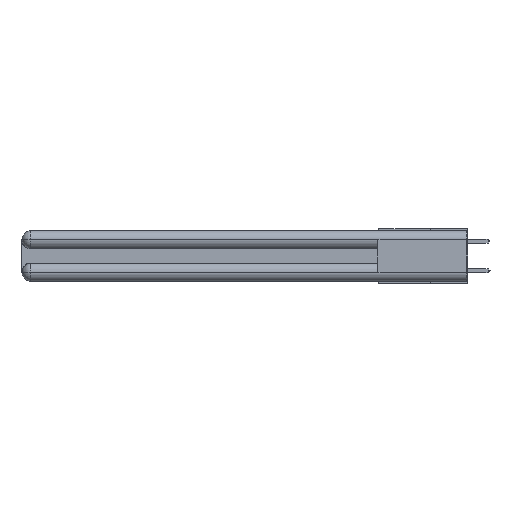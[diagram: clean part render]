
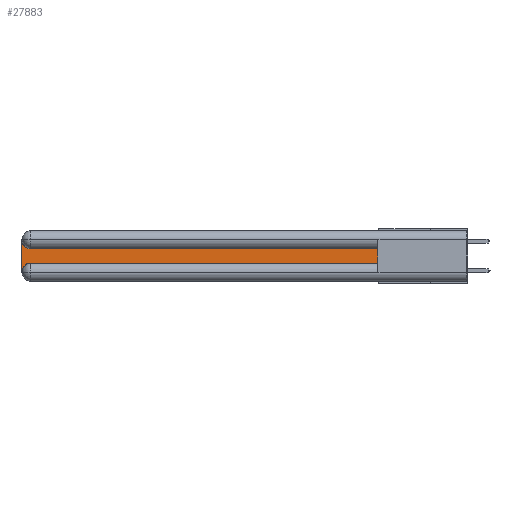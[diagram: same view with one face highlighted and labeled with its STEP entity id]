
A CAD part, left-side view. The second image highlights one B-rep face of the part: STEP entity #27883.
In plain terms, the highlighted planar face has unit normal (-1, 0, 0).
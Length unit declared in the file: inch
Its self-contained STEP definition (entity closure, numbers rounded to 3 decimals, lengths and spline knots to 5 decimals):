
#145 = EDGE_CURVE ( 'NONE', #4539, #19977, #30470, .T. ) ;
#1540 = DIRECTION ( 'NONE',  ( 0., 0., -1. ) ) ;
#2026 = EDGE_CURVE ( 'NONE', #13715, #15117, #4650, .T. ) ;
#3526 = VECTOR ( 'NONE', #26839, 39.37008 ) ;
#3580 = CARTESIAN_POINT ( 'NONE',  ( 0.075, 3., -0.2775 ) ) ;
#3583 = LINE ( 'NONE', #18115, #9339 ) ;
#3857 = ORIENTED_EDGE ( 'NONE', *, *, #10549, .T. ) ;
#4539 = VERTEX_POINT ( 'NONE', #18470 ) ;
#4556 = CARTESIAN_POINT ( 'NONE',  ( 0.075, 2.94, -0.2775 ) ) ;
#4650 = LINE ( 'NONE', #22990, #31207 ) ;
#4895 = DIRECTION ( 'NONE',  ( 0., -1., 0. ) ) ;
#5263 = FACE_OUTER_BOUND ( 'NONE', #29416, .T. ) ;
#6329 = AXIS2_PLACEMENT_3D ( 'NONE', #14744, #13019, #32342 ) ;
#7298 = VECTOR ( 'NONE', #19317, 39.37008 ) ;
#7432 = ORIENTED_EDGE ( 'NONE', *, *, #14962, .T. ) ;
#8144 = DIRECTION ( 'NONE',  ( 0., 0., 1. ) ) ;
#8427 = DIRECTION ( 'NONE',  ( 0., 0., -1. ) ) ;
#8766 = CARTESIAN_POINT ( 'NONE',  ( 0.075, 2.94, -0.0625 ) ) ;
#9339 = VECTOR ( 'NONE', #8144, 39.37008 ) ;
#10002 = CARTESIAN_POINT ( 'NONE',  ( 0.075, 2.94, -0.1225 ) ) ;
#10549 = EDGE_CURVE ( 'NONE', #31209, #11818, #31432, .T. ) ;
#10706 = CARTESIAN_POINT ( 'NONE',  ( 0.075, 2.94, -0.2175 ) ) ;
#11786 = CARTESIAN_POINT ( 'NONE',  ( 0.075, 3., -0.2175 ) ) ;
#11818 = VERTEX_POINT ( 'NONE', #10002 ) ;
#12960 = AXIS2_PLACEMENT_3D ( 'NONE', #4556, #14348, #1540 ) ;
#13019 = DIRECTION ( 'NONE',  ( 1., 0., 0. ) ) ;
#13715 = VERTEX_POINT ( 'NONE', #10706 ) ;
#13832 = DIRECTION ( 'NONE',  ( 1., 0., 0. ) ) ;
#14348 = DIRECTION ( 'NONE',  ( 1., 0., 0. ) ) ;
#14744 = CARTESIAN_POINT ( 'NONE',  ( 0.075, 3., -0.1225 ) ) ;
#14962 = EDGE_CURVE ( 'NONE', #11818, #4539, #27632, .T. ) ;
#15117 = VERTEX_POINT ( 'NONE', #22809 ) ;
#17193 = EDGE_CURVE ( 'NONE', #19977, #13715, #26908, .T. ) ;
#18115 = CARTESIAN_POINT ( 'NONE',  ( 0.075, 0.6, -0.2175 ) ) ;
#18470 = CARTESIAN_POINT ( 'NONE',  ( 0.075, 3., -0.0625 ) ) ;
#19317 = DIRECTION ( 'NONE',  ( 0., 1., 0. ) ) ;
#19977 = VERTEX_POINT ( 'NONE', #3580 ) ;
#21672 = CARTESIAN_POINT ( 'NONE',  ( 0.075, 0.6, -0.1225 ) ) ;
#22809 = CARTESIAN_POINT ( 'NONE',  ( 0.075, 0.6, -0.2175 ) ) ;
#22990 = CARTESIAN_POINT ( 'NONE',  ( 0.075, 0.6, -0.2175 ) ) ;
#23161 = ORIENTED_EDGE ( 'NONE', *, *, #28651, .T. ) ;
#24743 = PLANE ( 'NONE',  #6329 ) ;
#24983 = ORIENTED_EDGE ( 'NONE', *, *, #2026, .T. ) ;
#25610 = AXIS2_PLACEMENT_3D ( 'NONE', #8766, #13832, #8427 ) ;
#26839 = DIRECTION ( 'NONE',  ( 0., 0., -1. ) ) ;
#26908 = CIRCLE ( 'NONE', #12960, 0.06 ) ;
#27632 = CIRCLE ( 'NONE', #25610, 0.06 ) ;
#27883 = ADVANCED_FACE ( 'NONE', ( #5263 ), #24743, .F. ) ;
#28651 = EDGE_CURVE ( 'NONE', #15117, #31209, #3583, .T. ) ;
#29296 = CARTESIAN_POINT ( 'NONE',  ( 0.075, 0.6, -0.1225 ) ) ;
#29416 = EDGE_LOOP ( 'NONE', ( #3857, #7432, #33161, #33296, #24983, #23161 ) ) ;
#30470 = LINE ( 'NONE', #11786, #3526 ) ;
#31207 = VECTOR ( 'NONE', #4895, 39.37008 ) ;
#31209 = VERTEX_POINT ( 'NONE', #29296 ) ;
#31432 = LINE ( 'NONE', #21672, #7298 ) ;
#32342 = DIRECTION ( 'NONE',  ( 0., 0., -1. ) ) ;
#33161 = ORIENTED_EDGE ( 'NONE', *, *, #145, .T. ) ;
#33296 = ORIENTED_EDGE ( 'NONE', *, *, #17193, .T. ) ;
